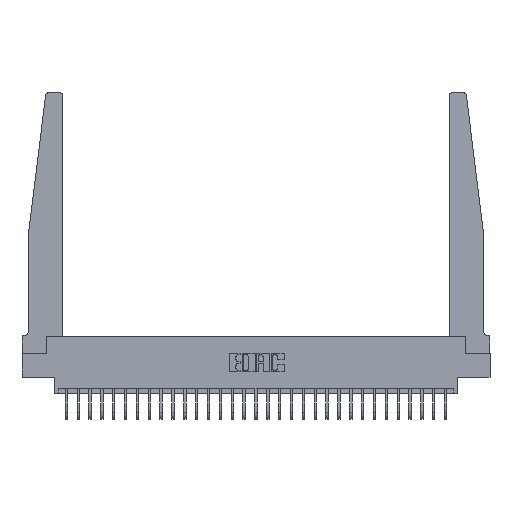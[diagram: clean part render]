
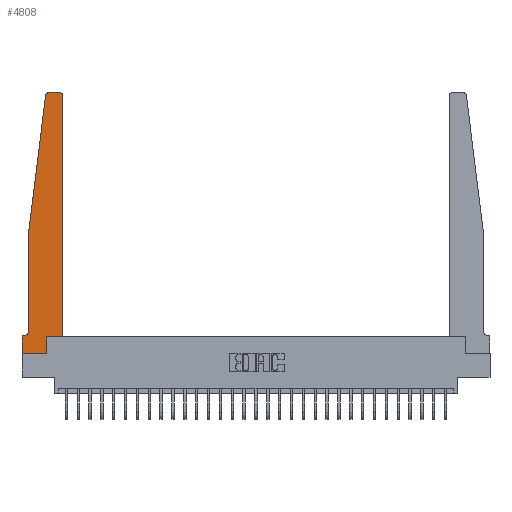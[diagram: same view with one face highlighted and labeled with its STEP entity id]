
A CAD part, top view. The second image highlights one B-rep face of the part: STEP entity #4808.
In plain terms, the highlighted planar face has unit normal (0, 0, 1).
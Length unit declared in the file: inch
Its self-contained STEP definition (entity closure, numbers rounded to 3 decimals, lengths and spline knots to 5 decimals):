
#185 = EDGE_CURVE ( 'NONE', #29278, #1324, #24781, .T. ) ;
#411 = ORIENTED_EDGE ( 'NONE', *, *, #13533, .T. ) ;
#426 = VECTOR ( 'NONE', #27130, 39.37008 ) ;
#734 = ORIENTED_EDGE ( 'NONE', *, *, #16554, .T. ) ;
#985 = LINE ( 'NONE', #24677, #1708 ) ;
#1320 = DIRECTION ( 'NONE',  ( -1., 0., 0. ) ) ;
#1324 = VERTEX_POINT ( 'NONE', #20776 ) ;
#1534 = LINE ( 'NONE', #3242, #13670 ) ;
#1631 = DIRECTION ( 'NONE',  ( 1., 0., 0. ) ) ;
#1708 = VECTOR ( 'NONE', #11035, 39.37008 ) ;
#1882 = CARTESIAN_POINT ( 'NONE',  ( 0.27653, 2.72, 0.37 ) ) ;
#2620 = VERTEX_POINT ( 'NONE', #24080 ) ;
#2958 = CARTESIAN_POINT ( 'NONE',  ( 0.2605, 0.18, 0.37 ) ) ;
#3242 = CARTESIAN_POINT ( 'NONE',  ( 0., 0., 0.37 ) ) ;
#3476 = CARTESIAN_POINT ( 'NONE',  ( 0., 0.1875, 0.37 ) ) ;
#3529 = VERTEX_POINT ( 'NONE', #5113 ) ;
#3697 = AXIS2_PLACEMENT_3D ( 'NONE', #10511, #24370, #1631 ) ;
#4083 = DIRECTION ( 'NONE',  ( 0., 0., 1. ) ) ;
#4115 = VERTEX_POINT ( 'NONE', #20234 ) ;
#4319 = ORIENTED_EDGE ( 'NONE', *, *, #18653, .T. ) ;
#4469 = EDGE_CURVE ( 'NONE', #22504, #23706, #985, .T. ) ;
#4523 = DIRECTION ( 'NONE',  ( -1., 0., 0. ) ) ;
#4808 = ADVANCED_FACE ( 'NONE', ( #12882 ), #7647, .T. ) ;
#5018 = EDGE_CURVE ( 'NONE', #14732, #23446, #28476, .T. ) ;
#5039 = ORIENTED_EDGE ( 'NONE', *, *, #185, .T. ) ;
#5113 = CARTESIAN_POINT ( 'NONE',  ( 0.24675, 2.72367, 0.37 ) ) ;
#5219 = DIRECTION ( 'NONE',  ( 1., 0., 0. ) ) ;
#5908 = EDGE_CURVE ( 'NONE', #1324, #14732, #18866, .T. ) ;
#6376 = DIRECTION ( 'NONE',  ( 1., 0., 0. ) ) ;
#6696 = CARTESIAN_POINT ( 'NONE',  ( 0.425, 2.72, 0.37 ) ) ;
#6762 = VECTOR ( 'NONE', #16448, 39.37008 ) ;
#7061 = EDGE_CURVE ( 'NONE', #4115, #7429, #11357, .T. ) ;
#7107 = DIRECTION ( 'NONE',  ( -1., 0., 0. ) ) ;
#7289 = CIRCLE ( 'NONE', #11770, 0.05 ) ;
#7429 = VERTEX_POINT ( 'NONE', #28137 ) ;
#7647 = PLANE ( 'NONE',  #24800 ) ;
#7930 = LINE ( 'NONE', #15649, #426 ) ;
#8002 = DIRECTION ( 'NONE',  ( 0., 0., -1. ) ) ;
#8214 = VERTEX_POINT ( 'NONE', #21723 ) ;
#8441 = CARTESIAN_POINT ( 'NONE',  ( 0.065, 1.25, 0.37 ) ) ;
#9021 = ORIENTED_EDGE ( 'NONE', *, *, #28478, .T. ) ;
#10109 = CARTESIAN_POINT ( 'NONE',  ( 0.015, 0.2375, 0.37 ) ) ;
#10511 = CARTESIAN_POINT ( 'NONE',  ( 0.395, 2.72, 0.37 ) ) ;
#10552 = CIRCLE ( 'NONE', #3697, 0.03 ) ;
#10899 = VECTOR ( 'NONE', #4523, 39.37008 ) ;
#11035 = DIRECTION ( 'NONE',  ( 0., -1., 0. ) ) ;
#11357 = LINE ( 'NONE', #22407, #15626 ) ;
#11770 = AXIS2_PLACEMENT_3D ( 'NONE', #10109, #8002, #1320 ) ;
#12798 = VECTOR ( 'NONE', #29136, 39.37008 ) ;
#12812 = EDGE_CURVE ( 'NONE', #23446, #4115, #10552, .T. ) ;
#12882 = FACE_OUTER_BOUND ( 'NONE', #18659, .T. ) ;
#12932 = ORIENTED_EDGE ( 'NONE', *, *, #7061, .T. ) ;
#13108 = CARTESIAN_POINT ( 'NONE',  ( 0., 0., 0.37 ) ) ;
#13533 = EDGE_CURVE ( 'NONE', #23706, #29278, #1534, .T. ) ;
#13670 = VECTOR ( 'NONE', #5219, 39.37008 ) ;
#14393 = DIRECTION ( 'NONE',  ( 0., 1., 0. ) ) ;
#14726 = DIRECTION ( 'NONE',  ( 1., 0., 0. ) ) ;
#14732 = VERTEX_POINT ( 'NONE', #26765 ) ;
#15203 = LINE ( 'NONE', #8441, #24510 ) ;
#15626 = VECTOR ( 'NONE', #7107, 39.37008 ) ;
#15649 = CARTESIAN_POINT ( 'NONE',  ( 0.065, 1.25, 0.37 ) ) ;
#15794 = CARTESIAN_POINT ( 'NONE',  ( 0.2605, 0., 0.37 ) ) ;
#16448 = DIRECTION ( 'NONE',  ( 1., 0., 0. ) ) ;
#16477 = ORIENTED_EDGE ( 'NONE', *, *, #16726, .T. ) ;
#16554 = EDGE_CURVE ( 'NONE', #27752, #2620, #7289, .T. ) ;
#16726 = EDGE_CURVE ( 'NONE', #2620, #22504, #19077, .T. ) ;
#17507 = AXIS2_PLACEMENT_3D ( 'NONE', #1882, #4083, #6376 ) ;
#17791 = EDGE_CURVE ( 'NONE', #8214, #27752, #15203, .T. ) ;
#18186 = ORIENTED_EDGE ( 'NONE', *, *, #5908, .T. ) ;
#18653 = EDGE_CURVE ( 'NONE', #7429, #3529, #19005, .T. ) ;
#18659 = EDGE_LOOP ( 'NONE', ( #12932, #4319, #9021, #24553, #734, #16477, #26787, #411, #5039, #18186, #19692, #27854 ) ) ;
#18866 = LINE ( 'NONE', #25719, #6762 ) ;
#19005 = CIRCLE ( 'NONE', #17507, 0.03 ) ;
#19077 = LINE ( 'NONE', #25734, #10899 ) ;
#19692 = ORIENTED_EDGE ( 'NONE', *, *, #5018, .T. ) ;
#20234 = CARTESIAN_POINT ( 'NONE',  ( 0.395, 2.75, 0.37 ) ) ;
#20776 = CARTESIAN_POINT ( 'NONE',  ( 0.2605, 0.18, 0.37 ) ) ;
#21723 = CARTESIAN_POINT ( 'NONE',  ( 0.065, 1.25, 0.37 ) ) ;
#22407 = CARTESIAN_POINT ( 'NONE',  ( 0.25, 2.75, 0.37 ) ) ;
#22504 = VERTEX_POINT ( 'NONE', #3476 ) ;
#22705 = DIRECTION ( 'NONE',  ( 0., -1., 0. ) ) ;
#23446 = VERTEX_POINT ( 'NONE', #6696 ) ;
#23706 = VERTEX_POINT ( 'NONE', #13108 ) ;
#23711 = VECTOR ( 'NONE', #14393, 39.37008 ) ;
#24080 = CARTESIAN_POINT ( 'NONE',  ( 0.015, 0.1875, 0.37 ) ) ;
#24370 = DIRECTION ( 'NONE',  ( 0., 0., 1. ) ) ;
#24377 = CARTESIAN_POINT ( 'NONE',  ( 0.065, 0.2375, 0.37 ) ) ;
#24510 = VECTOR ( 'NONE', #22705, 39.37008 ) ;
#24553 = ORIENTED_EDGE ( 'NONE', *, *, #17791, .T. ) ;
#24677 = CARTESIAN_POINT ( 'NONE',  ( 0., 0., 0.37 ) ) ;
#24781 = LINE ( 'NONE', #2958, #23711 ) ;
#24800 = AXIS2_PLACEMENT_3D ( 'NONE', #28061, #25880, #14726 ) ;
#25719 = CARTESIAN_POINT ( 'NONE',  ( 0.425, 0.18, 0.37 ) ) ;
#25734 = CARTESIAN_POINT ( 'NONE',  ( 0.065, 0.1875, 0.37 ) ) ;
#25880 = DIRECTION ( 'NONE',  ( 0., 0., 1. ) ) ;
#26765 = CARTESIAN_POINT ( 'NONE',  ( 0.425, 0.18, 0.37 ) ) ;
#26787 = ORIENTED_EDGE ( 'NONE', *, *, #4469, .T. ) ;
#26791 = CARTESIAN_POINT ( 'NONE',  ( 0.425, 0.18, 0.37 ) ) ;
#27130 = DIRECTION ( 'NONE',  ( -0.122, -0.992, 0. ) ) ;
#27752 = VERTEX_POINT ( 'NONE', #24377 ) ;
#27854 = ORIENTED_EDGE ( 'NONE', *, *, #12812, .T. ) ;
#28061 = CARTESIAN_POINT ( 'NONE',  ( 0., 0.1875, 0.37 ) ) ;
#28137 = CARTESIAN_POINT ( 'NONE',  ( 0.27653, 2.75, 0.37 ) ) ;
#28476 = LINE ( 'NONE', #26791, #12798 ) ;
#28478 = EDGE_CURVE ( 'NONE', #3529, #8214, #7930, .T. ) ;
#29136 = DIRECTION ( 'NONE',  ( 0., 1., 0. ) ) ;
#29278 = VERTEX_POINT ( 'NONE', #15794 ) ;
